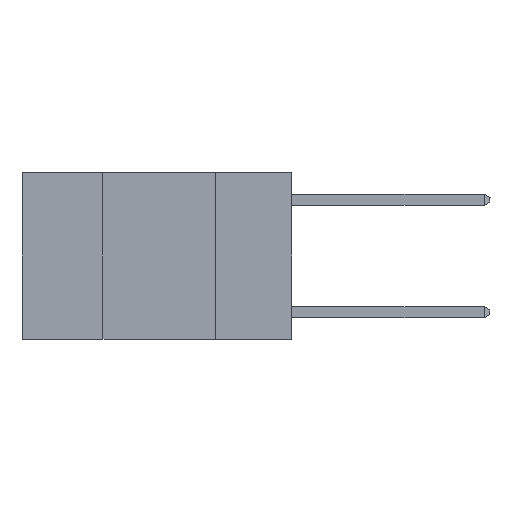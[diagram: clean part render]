
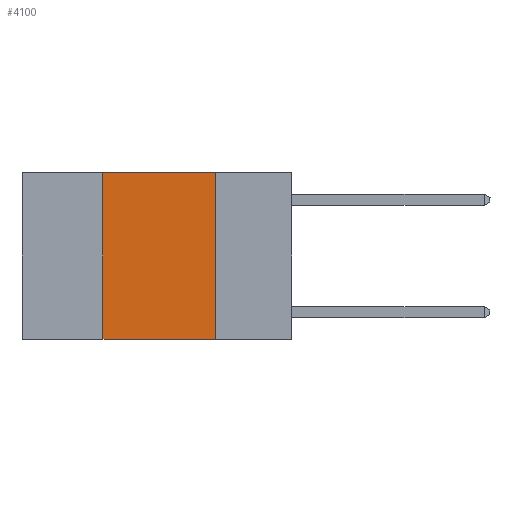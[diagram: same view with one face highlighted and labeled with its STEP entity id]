
A CAD part, left-side view. The second image highlights one B-rep face of the part: STEP entity #4100.
In plain terms, the highlighted planar face has unit normal (-1, 0, 0).
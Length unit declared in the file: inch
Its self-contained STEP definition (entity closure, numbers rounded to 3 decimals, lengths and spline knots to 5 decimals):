
#476 = LINE ( 'NONE', #12627, #3005 ) ;
#942 = DIRECTION ( 'NONE',  ( 0., 0., -1. ) ) ;
#1387 = CARTESIAN_POINT ( 'NONE',  ( 0., 0.42, -0.37 ) ) ;
#2202 = ORIENTED_EDGE ( 'NONE', *, *, #16550, .F. ) ;
#3005 = VECTOR ( 'NONE', #11092, 39.37008 ) ;
#3487 = CARTESIAN_POINT ( 'NONE',  ( 0., 0.17, 0. ) ) ;
#3726 = CARTESIAN_POINT ( 'NONE',  ( 0., 0.42, 0. ) ) ;
#4100 = ADVANCED_FACE ( 'NONE', ( #4306 ), #11815, .F. ) ;
#4134 = EDGE_CURVE ( 'NONE', #18370, #18120, #11698, .T. ) ;
#4306 = FACE_OUTER_BOUND ( 'NONE', #7469, .T. ) ;
#4863 = CARTESIAN_POINT ( 'NONE',  ( 0., 0.17, 0. ) ) ;
#6056 = VERTEX_POINT ( 'NONE', #13427 ) ;
#7469 = EDGE_LOOP ( 'NONE', ( #2202, #20198, #14366, #11628 ) ) ;
#10069 = CARTESIAN_POINT ( 'NONE',  ( 0., 0.42, 0. ) ) ;
#10256 = VECTOR ( 'NONE', #22764, 39.37008 ) ;
#11059 = VECTOR ( 'NONE', #19186, 39.37008 ) ;
#11092 = DIRECTION ( 'NONE',  ( 0., -1., 0. ) ) ;
#11341 = CARTESIAN_POINT ( 'NONE',  ( 0., 0.6, 0. ) ) ;
#11628 = ORIENTED_EDGE ( 'NONE', *, *, #18138, .T. ) ;
#11698 = LINE ( 'NONE', #10069, #10256 ) ;
#11815 = PLANE ( 'NONE',  #22386 ) ;
#12418 = VECTOR ( 'NONE', #17974, 39.37008 ) ;
#12627 = CARTESIAN_POINT ( 'NONE',  ( 0., 0.6, -0.37 ) ) ;
#13316 = DIRECTION ( 'NONE',  ( 1., 0., 0. ) ) ;
#13427 = CARTESIAN_POINT ( 'NONE',  ( 0., 0.17, -0.37 ) ) ;
#14366 = ORIENTED_EDGE ( 'NONE', *, *, #4134, .F. ) ;
#14382 = CARTESIAN_POINT ( 'NONE',  ( 0., 0.6, 0. ) ) ;
#15782 = EDGE_CURVE ( 'NONE', #18120, #20568, #18073, .T. ) ;
#16550 = EDGE_CURVE ( 'NONE', #20568, #6056, #20685, .T. ) ;
#17974 = DIRECTION ( 'NONE',  ( 0., -1., 0. ) ) ;
#18073 = LINE ( 'NONE', #14382, #12418 ) ;
#18120 = VERTEX_POINT ( 'NONE', #3726 ) ;
#18138 = EDGE_CURVE ( 'NONE', #18370, #6056, #476, .T. ) ;
#18370 = VERTEX_POINT ( 'NONE', #1387 ) ;
#19186 = DIRECTION ( 'NONE',  ( 0., 0., -1. ) ) ;
#20198 = ORIENTED_EDGE ( 'NONE', *, *, #15782, .F. ) ;
#20568 = VERTEX_POINT ( 'NONE', #3487 ) ;
#20685 = LINE ( 'NONE', #4863, #11059 ) ;
#22386 = AXIS2_PLACEMENT_3D ( 'NONE', #11341, #13316, #942 ) ;
#22764 = DIRECTION ( 'NONE',  ( 0., 0., 1. ) ) ;
